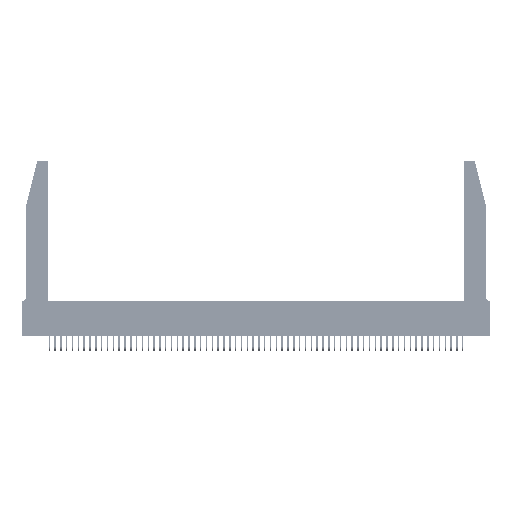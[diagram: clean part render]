
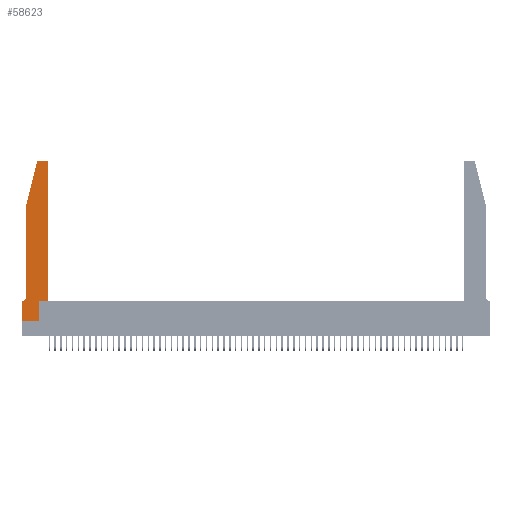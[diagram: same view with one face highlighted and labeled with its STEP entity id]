
A CAD part, top view. The second image highlights one B-rep face of the part: STEP entity #58623.
In plain terms, the highlighted planar face has unit normal (0, 0, 1).
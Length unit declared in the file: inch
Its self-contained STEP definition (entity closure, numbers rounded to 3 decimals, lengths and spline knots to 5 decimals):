
#386 = DIRECTION ( 'NONE',  ( 0., 0., 1. ) ) ;
#849 = VERTEX_POINT ( 'NONE', #11260 ) ;
#1965 = AXIS2_PLACEMENT_3D ( 'NONE', #13385, #39348, #58243 ) ;
#2813 = ORIENTED_EDGE ( 'NONE', *, *, #44482, .T. ) ;
#3230 = CARTESIAN_POINT ( 'NONE',  ( 0.4505, 0.35, 0.37 ) ) ;
#3626 = DIRECTION ( 'NONE',  ( 0., -1., 0. ) ) ;
#4620 = AXIS2_PLACEMENT_3D ( 'NONE', #14214, #46402, #55199 ) ;
#4656 = LINE ( 'NONE', #16768, #40935 ) ;
#4845 = AXIS2_PLACEMENT_3D ( 'NONE', #45128, #44923, #54099 ) ;
#6690 = VERTEX_POINT ( 'NONE', #33915 ) ;
#7882 = VERTEX_POINT ( 'NONE', #48081 ) ;
#8125 = VERTEX_POINT ( 'NONE', #58417 ) ;
#9458 = CARTESIAN_POINT ( 'NONE',  ( 0.4505, 0.35, 0.37 ) ) ;
#9668 = LINE ( 'NONE', #33441, #15357 ) ;
#11260 = CARTESIAN_POINT ( 'NONE',  ( 0.284, 2.75, 0.37 ) ) ;
#11884 = LINE ( 'NONE', #26708, #50333 ) ;
#12545 = CARTESIAN_POINT ( 'NONE',  ( 0.0055, 0.35, 0.37 ) ) ;
#13128 = VECTOR ( 'NONE', #39636, 39.37008 ) ;
#13159 = CARTESIAN_POINT ( 'NONE',  ( 0.0755, 2., 0.37 ) ) ;
#13385 = CARTESIAN_POINT ( 'NONE',  ( 0., 0.35, 0.37 ) ) ;
#13452 = CARTESIAN_POINT ( 'NONE',  ( 0.4505, 2.72, 0.37 ) ) ;
#14214 = CARTESIAN_POINT ( 'NONE',  ( 0.284, 2.72, 0.37 ) ) ;
#15357 = VECTOR ( 'NONE', #51930, 39.37008 ) ;
#15732 = VECTOR ( 'NONE', #38103, 39.37008 ) ;
#15860 = ORIENTED_EDGE ( 'NONE', *, *, #42318, .T. ) ;
#16768 = CARTESIAN_POINT ( 'NONE',  ( 0.2865, 0.35, 0.37 ) ) ;
#17048 = VERTEX_POINT ( 'NONE', #30163 ) ;
#17445 = EDGE_CURVE ( 'NONE', #849, #8125, #58401, .T. ) ;
#18448 = ORIENTED_EDGE ( 'NONE', *, *, #54411, .T. ) ;
#18572 = ORIENTED_EDGE ( 'NONE', *, *, #39916, .T. ) ;
#18716 = EDGE_CURVE ( 'NONE', #7882, #6690, #4656, .T. ) ;
#18945 = FACE_OUTER_BOUND ( 'NONE', #33037, .T. ) ;
#19781 = LINE ( 'NONE', #3230, #54672 ) ;
#20529 = DIRECTION ( 'NONE',  ( 0., 1., 0. ) ) ;
#20723 = VECTOR ( 'NONE', #24034, 39.37008 ) ;
#21577 = VERTEX_POINT ( 'NONE', #49710 ) ;
#21858 = ORIENTED_EDGE ( 'NONE', *, *, #57804, .T. ) ;
#22200 = DIRECTION ( 'NONE',  ( -1., 0., 0. ) ) ;
#23224 = VECTOR ( 'NONE', #49986, 39.37008 ) ;
#23333 = CARTESIAN_POINT ( 'NONE',  ( 0.4505, 0.35, 0.37 ) ) ;
#24000 = VERTEX_POINT ( 'NONE', #13159 ) ;
#24034 = DIRECTION ( 'NONE',  ( 0., -1., 0. ) ) ;
#24646 = LINE ( 'NONE', #23333, #23224 ) ;
#25115 = VECTOR ( 'NONE', #22200, 39.37008 ) ;
#25254 = LINE ( 'NONE', #39247, #13128 ) ;
#26147 = VERTEX_POINT ( 'NONE', #34602 ) ;
#26708 = CARTESIAN_POINT ( 'NONE',  ( 0.0755, 2., 0.37 ) ) ;
#27519 = EDGE_CURVE ( 'NONE', #37694, #55609, #19781, .T. ) ;
#27598 = EDGE_CURVE ( 'NONE', #24000, #21577, #11884, .T. ) ;
#27633 = VERTEX_POINT ( 'NONE', #12545 ) ;
#27653 = CARTESIAN_POINT ( 'NONE',  ( 0.4205, 2.72, 0.37 ) ) ;
#29703 = ORIENTED_EDGE ( 'NONE', *, *, #51387, .T. ) ;
#30163 = CARTESIAN_POINT ( 'NONE',  ( 0.4205, 2.75, 0.37 ) ) ;
#31499 = ORIENTED_EDGE ( 'NONE', *, *, #33005, .T. ) ;
#32216 = ORIENTED_EDGE ( 'NONE', *, *, #27519, .T. ) ;
#33005 = EDGE_CURVE ( 'NONE', #8125, #24000, #38510, .T. ) ;
#33037 = EDGE_LOOP ( 'NONE', ( #18572, #47066, #31499, #44732, #15860, #2813, #44972, #21858, #34583, #18448, #32216, #29703 ) ) ;
#33441 = CARTESIAN_POINT ( 'NONE',  ( 0., 0., 0.37 ) ) ;
#33527 = CARTESIAN_POINT ( 'NONE',  ( 0.0755, 2., 0.37 ) ) ;
#33915 = CARTESIAN_POINT ( 'NONE',  ( 0.2865, 0.35, 0.37 ) ) ;
#34484 = DIRECTION ( 'NONE',  ( 0., 1., 0. ) ) ;
#34583 = ORIENTED_EDGE ( 'NONE', *, *, #18716, .T. ) ;
#34602 = CARTESIAN_POINT ( 'NONE',  ( 0., 0.35, 0.37 ) ) ;
#36972 = DIRECTION ( 'NONE',  ( 1., 0., 0. ) ) ;
#37694 = VERTEX_POINT ( 'NONE', #9458 ) ;
#38103 = DIRECTION ( 'NONE',  ( -0.239, -0.971, 0. ) ) ;
#38510 = LINE ( 'NONE', #33527, #15732 ) ;
#39247 = CARTESIAN_POINT ( 'NONE',  ( 0.2605, 2.75, 0.37 ) ) ;
#39348 = DIRECTION ( 'NONE',  ( 0., 0., 1. ) ) ;
#39636 = DIRECTION ( 'NONE',  ( -1., 0., 0. ) ) ;
#39916 = EDGE_CURVE ( 'NONE', #17048, #849, #25254, .T. ) ;
#39963 = CIRCLE ( 'NONE', #55789, 0.03 ) ;
#40011 = PLANE ( 'NONE',  #1965 ) ;
#40935 = VECTOR ( 'NONE', #34484, 39.37008 ) ;
#41771 = VERTEX_POINT ( 'NONE', #45591 ) ;
#42318 = EDGE_CURVE ( 'NONE', #21577, #27633, #53476, .T. ) ;
#42478 = EDGE_CURVE ( 'NONE', #26147, #41771, #43482, .T. ) ;
#43482 = LINE ( 'NONE', #51285, #20723 ) ;
#44482 = EDGE_CURVE ( 'NONE', #27633, #26147, #49280, .T. ) ;
#44732 = ORIENTED_EDGE ( 'NONE', *, *, #27598, .T. ) ;
#44923 = DIRECTION ( 'NONE',  ( 0., 0., -1. ) ) ;
#44972 = ORIENTED_EDGE ( 'NONE', *, *, #42478, .T. ) ;
#45128 = CARTESIAN_POINT ( 'NONE',  ( 0.0055, 0.42, 0.37 ) ) ;
#45591 = CARTESIAN_POINT ( 'NONE',  ( 0., 0., 0.37 ) ) ;
#46402 = DIRECTION ( 'NONE',  ( 0., 0., 1. ) ) ;
#47066 = ORIENTED_EDGE ( 'NONE', *, *, #17445, .T. ) ;
#48081 = CARTESIAN_POINT ( 'NONE',  ( 0.2865, 0., 0.37 ) ) ;
#49280 = LINE ( 'NONE', #49444, #25115 ) ;
#49444 = CARTESIAN_POINT ( 'NONE',  ( 0.0755, 0.35, 0.37 ) ) ;
#49710 = CARTESIAN_POINT ( 'NONE',  ( 0.0755, 0.42, 0.37 ) ) ;
#49986 = DIRECTION ( 'NONE',  ( 1., 0., 0. ) ) ;
#50333 = VECTOR ( 'NONE', #3626, 39.37008 ) ;
#51285 = CARTESIAN_POINT ( 'NONE',  ( 0., 0., 0.37 ) ) ;
#51387 = EDGE_CURVE ( 'NONE', #55609, #17048, #39963, .T. ) ;
#51930 = DIRECTION ( 'NONE',  ( 1., 0., 0. ) ) ;
#53476 = CIRCLE ( 'NONE', #4845, 0.07 ) ;
#54099 = DIRECTION ( 'NONE',  ( -1., 0., 0. ) ) ;
#54411 = EDGE_CURVE ( 'NONE', #6690, #37694, #24646, .T. ) ;
#54672 = VECTOR ( 'NONE', #20529, 39.37008 ) ;
#55199 = DIRECTION ( 'NONE',  ( 1., 0., 0. ) ) ;
#55609 = VERTEX_POINT ( 'NONE', #13452 ) ;
#55789 = AXIS2_PLACEMENT_3D ( 'NONE', #27653, #386, #36972 ) ;
#57804 = EDGE_CURVE ( 'NONE', #41771, #7882, #9668, .T. ) ;
#58243 = DIRECTION ( 'NONE',  ( 1., 0., 0. ) ) ;
#58401 = CIRCLE ( 'NONE', #4620, 0.03 ) ;
#58417 = CARTESIAN_POINT ( 'NONE',  ( 0.25487, 2.72718, 0.37 ) ) ;
#58623 = ADVANCED_FACE ( 'NONE', ( #18945 ), #40011, .T. ) ;
